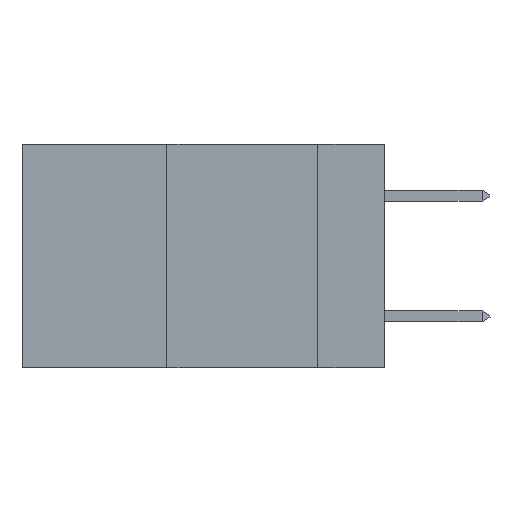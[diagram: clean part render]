
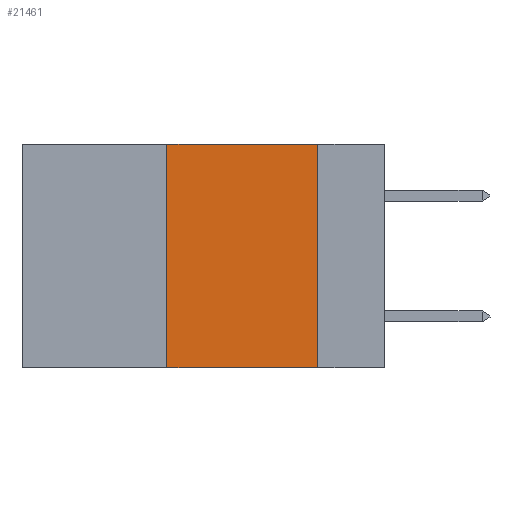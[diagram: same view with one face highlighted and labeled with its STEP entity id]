
A CAD part, left-side view. The second image highlights one B-rep face of the part: STEP entity #21461.
In plain terms, the highlighted planar face has unit normal (-1, 0, 0).
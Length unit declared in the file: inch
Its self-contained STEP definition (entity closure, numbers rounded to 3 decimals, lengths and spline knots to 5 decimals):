
#225 = ORIENTED_EDGE ( 'NONE', *, *, #17025, .F. ) ;
#391 = VERTEX_POINT ( 'NONE', #6978 ) ;
#1775 = DIRECTION ( 'NONE',  ( 0., 0., 1. ) ) ;
#3035 = VECTOR ( 'NONE', #18667, 39.37008 ) ;
#3266 = EDGE_CURVE ( 'NONE', #7530, #391, #8835, .T. ) ;
#4070 = VECTOR ( 'NONE', #22260, 39.37008 ) ;
#6105 = CARTESIAN_POINT ( 'NONE',  ( 0., 0.11, 0. ) ) ;
#6430 = VECTOR ( 'NONE', #1775, 39.37008 ) ;
#6727 = ORIENTED_EDGE ( 'NONE', *, *, #18662, .T. ) ;
#6978 = CARTESIAN_POINT ( 'NONE',  ( 0., 0.11, 0. ) ) ;
#7530 = VERTEX_POINT ( 'NONE', #13761 ) ;
#7700 = LINE ( 'NONE', #14275, #21401 ) ;
#8030 = LINE ( 'NONE', #6105, #3035 ) ;
#8438 = CARTESIAN_POINT ( 'NONE',  ( 0., 0.11, -0.37 ) ) ;
#8575 = CARTESIAN_POINT ( 'NONE',  ( 0., 0.36, -0.37 ) ) ;
#8835 = LINE ( 'NONE', #18711, #4070 ) ;
#8874 = FACE_OUTER_BOUND ( 'NONE', #13241, .T. ) ;
#10406 = ORIENTED_EDGE ( 'NONE', *, *, #3266, .F. ) ;
#10759 = CARTESIAN_POINT ( 'NONE',  ( 0., 0.36, 0. ) ) ;
#10777 = VERTEX_POINT ( 'NONE', #8575 ) ;
#11066 = DIRECTION ( 'NONE',  ( 0., 0., -1. ) ) ;
#11469 = EDGE_CURVE ( 'NONE', #10777, #7530, #15398, .T. ) ;
#12496 = DIRECTION ( 'NONE',  ( 0., -1., 0. ) ) ;
#13241 = EDGE_LOOP ( 'NONE', ( #225, #10406, #19900, #6727 ) ) ;
#13761 = CARTESIAN_POINT ( 'NONE',  ( 0., 0.36, 0. ) ) ;
#14275 = CARTESIAN_POINT ( 'NONE',  ( 0., 0.6, -0.37 ) ) ;
#15398 = LINE ( 'NONE', #10759, #6430 ) ;
#15547 = VERTEX_POINT ( 'NONE', #8438 ) ;
#16394 = PLANE ( 'NONE',  #19521 ) ;
#17025 = EDGE_CURVE ( 'NONE', #391, #15547, #8030, .T. ) ;
#18662 = EDGE_CURVE ( 'NONE', #10777, #15547, #7700, .T. ) ;
#18667 = DIRECTION ( 'NONE',  ( 0., 0., -1. ) ) ;
#18711 = CARTESIAN_POINT ( 'NONE',  ( 0., 0.6, 0. ) ) ;
#19521 = AXIS2_PLACEMENT_3D ( 'NONE', #19958, #21735, #11066 ) ;
#19900 = ORIENTED_EDGE ( 'NONE', *, *, #11469, .F. ) ;
#19958 = CARTESIAN_POINT ( 'NONE',  ( 0., 0.6, 0. ) ) ;
#21401 = VECTOR ( 'NONE', #12496, 39.37008 ) ;
#21461 = ADVANCED_FACE ( 'NONE', ( #8874 ), #16394, .F. ) ;
#21735 = DIRECTION ( 'NONE',  ( 1., 0., 0. ) ) ;
#22260 = DIRECTION ( 'NONE',  ( 0., -1., 0. ) ) ;
